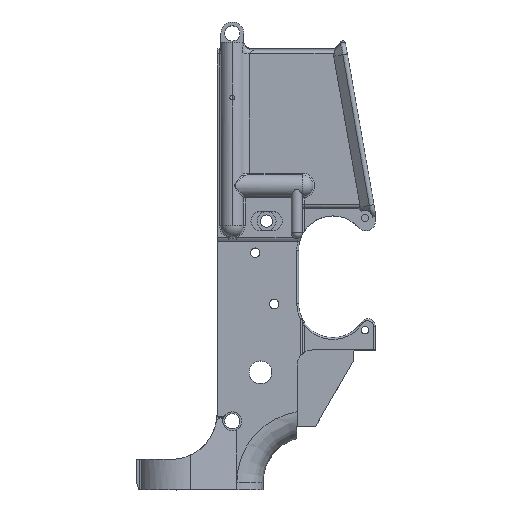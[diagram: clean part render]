
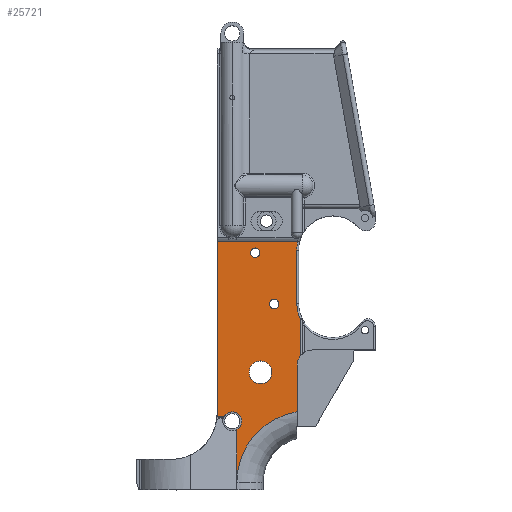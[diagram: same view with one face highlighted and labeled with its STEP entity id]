
A CAD part, top view. The second image highlights one B-rep face of the part: STEP entity #25721.
In plain terms, the highlighted planar face has unit normal (0, 0, 1).
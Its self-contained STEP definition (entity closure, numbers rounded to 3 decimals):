
#3836=CARTESIAN_POINT(' ',(0.033,-0.451,0.045));
#3837=VERTEX_POINT(' ',#3836);
#3926=CARTESIAN_POINT(' ',(0.033,-0.451,0.045));
#3931=DIRECTION(' ',(0.,1.,0.));
#3936=VECTOR(' ',#3931,1.);
#3941=LINE('',#3926,#3936);
#3946=CARTESIAN_POINT(' ',(0.033,-0.364,0.045));
#3947=VERTEX_POINT(' ',#3946);
#3951=EDGE_CURVE(' ',#3837,#3947,#3941,.T.);
#13861=CARTESIAN_POINT(' ',(0.,-0.338,0.045));
#13862=VERTEX_POINT(' ',#13861);
#13876=CARTESIAN_POINT(' ',(0.,-0.338,0.045));
#13881=DIRECTION(' ',(0.,1.,0.));
#13886=VECTOR(' ',#13881,1.);
#13891=LINE('',#13876,#13886);
#13896=CARTESIAN_POINT(' ',(0.,-0.055,0.045));
#13897=VERTEX_POINT(' ',#13896);
#13901=EDGE_CURVE(' ',#13862,#13897,#13891,.T.);
#17491=CARTESIAN_POINT(' ',(0.,-0.342,0.045));
#17492=VERTEX_POINT(' ',#17491);
#17506=CARTESIAN_POINT(' ',(-0.075,-0.338,0.045));
#17511=DIRECTION(' ',(0.,0.,1.));
#17516=DIRECTION(' ',(0.999,-0.053,0.));
#17521=AXIS2_PLACEMENT_3D(' ',#17506,#17511,#17516);
#17526=CIRCLE('',#17521,0.075);
#17531=EDGE_CURVE(' ',#17492,#13862,#17526,.T.);
#17851=CARTESIAN_POINT(' ',(0.041,-0.35,0.045));
#17852=VERTEX_POINT(' ',#17851);
#17866=CARTESIAN_POINT(' ',(0.025,-0.35,0.045));
#17871=DIRECTION(' ',(0.,0.,1.));
#17876=DIRECTION(' ',(1.,0.,0.));
#17881=AXIS2_PLACEMENT_3D(' ',#17866,#17871,#17876);
#17886=CIRCLE('',#17881,0.016);
#17891=CARTESIAN_POINT(' ',(0.011,-0.342,0.045));
#17892=VERTEX_POINT(' ',#17891);
#17896=EDGE_CURVE(' ',#17852,#17892,#17886,.T.);
#18146=CARTESIAN_POINT(' ',(0.025,-0.35,0.045));
#18151=DIRECTION(' ',(0.,0.,1.));
#18156=DIRECTION(' ',(0.481,-0.877,0.));
#18161=AXIS2_PLACEMENT_3D(' ',#18146,#18151,#18156);
#18166=CIRCLE('',#18161,0.016);
#18171=EDGE_CURVE(' ',#3947,#17852,#18166,.T.);
#24946=CARTESIAN_POINT(' ',(0.132,-0.334,0.045));
#24947=VERTEX_POINT(' ',#24946);
#24961=CARTESIAN_POINT(' ',(0.132,-0.334,0.045));
#24966=CARTESIAN_POINT(' ',(0.125,-0.336,0.045));
#24971=CARTESIAN_POINT(' ',(0.118,-0.337,0.045));
#24976=CARTESIAN_POINT(' ',(0.103,-0.342,0.045));
#24981=CARTESIAN_POINT(' ',(0.095,-0.347,0.045));
#24986=CARTESIAN_POINT(' ',(0.081,-0.355,0.045));
#24991=CARTESIAN_POINT(' ',(0.076,-0.359,0.045));
#24996=CARTESIAN_POINT(' ',(0.067,-0.367,0.045));
#25001=CARTESIAN_POINT(' ',(0.065,-0.37,0.045));
#25006=CARTESIAN_POINT(' ',(0.06,-0.375,0.045));
#25011=CARTESIAN_POINT(' ',(0.058,-0.377,0.045));
#25016=CARTESIAN_POINT(' ',(0.054,-0.382,0.045));
#25021=CARTESIAN_POINT(' ',(0.052,-0.385,0.045));
#25026=CARTESIAN_POINT(' ',(0.046,-0.396,0.045));
#25031=CARTESIAN_POINT(' ',(0.043,-0.402,0.045));
#25036=CARTESIAN_POINT(' ',(0.039,-0.412,0.045));
#25041=CARTESIAN_POINT(' ',(0.038,-0.416,0.045));
#25046=CARTESIAN_POINT(' ',(0.034,-0.43,0.045));
#25051=CARTESIAN_POINT(' ',(0.033,-0.435,0.045));
#25056=CARTESIAN_POINT(' ',(0.033,-0.442,0.045));
#25061=CARTESIAN_POINT(' ',(0.033,-0.445,0.045));
#25066=CARTESIAN_POINT(' ',(0.033,-0.451,0.045));
#25071=B_SPLINE_CURVE_WITH_KNOTS('',3,(#24961,#24966,#24971,#24976,#24981,#24986,#24991,#24996,#25001,#25006,#25011,#25016,#25021,#25026,#25031,#25036,#25041,#25046,#25051,#25056,#25061,#25066),.UNSPECIFIED.,.F.,.U.,(4,2,2,2,2,2,2,2,2,2,4),(0.,0.1,0.22,0.3,0.396,0.496,0.596,0.696,0.796,0.916,1.),.UNSPECIFIED.);
#25076=EDGE_CURVE(' ',#24947,#3837,#25071,.T.);
#25101=DIRECTION(' ',(0.,0.,1.));
#25106=CARTESIAN_POINT(' ',(0.,-0.451,0.045));
#25111=DIRECTION(' ',(1.,0.,0.));
#25116=AXIS2_PLACEMENT_3D(' ',#25106,#25101,#25111);
#25121=PLANE('',#25116);
#25126=ORIENTED_EDGE(' ',*,*,#17531,.F.);
#25131=CARTESIAN_POINT(' ',(0.,-0.342,0.045));
#25136=DIRECTION(' ',(0.997,-0.077,0.));
#25141=VECTOR(' ',#25136,1.);
#25146=LINE('',#25131,#25141);
#25151=EDGE_CURVE(' ',#17492,#17892,#25146,.T.);
#25156=ORIENTED_EDGE(' ',*,*,#25151,.T.);
#25161=ORIENTED_EDGE(' ',*,*,#17896,.F.);
#25166=ORIENTED_EDGE(' ',*,*,#18171,.F.);
#25171=ORIENTED_EDGE(' ',*,*,#3951,.F.);
#25176=ORIENTED_EDGE(' ',*,*,#25076,.F.);
#25181=CARTESIAN_POINT(' ',(0.132,-0.334,0.045));
#25186=DIRECTION(' ',(0.,1.,0.));
#25191=VECTOR(' ',#25186,1.);
#25196=LINE('',#25181,#25191);
#25201=CARTESIAN_POINT(' ',(0.132,-0.258,0.045));
#25202=VERTEX_POINT(' ',#25201);
#25206=EDGE_CURVE(' ',#24947,#25202,#25196,.T.);
#25211=ORIENTED_EDGE(' ',*,*,#25206,.T.);
#25216=CARTESIAN_POINT(' ',(0.157,-0.258,0.045));
#25221=DIRECTION(' ',(0.,0.,-1.));
#25226=DIRECTION(' ',(-1.,0.,0.));
#25231=AXIS2_PLACEMENT_3D(' ',#25216,#25221,#25226);
#25236=CIRCLE('',#25231,0.025);
#25241=CARTESIAN_POINT(' ',(0.137,-0.242,0.045));
#25242=VERTEX_POINT(' ',#25241);
#25246=EDGE_CURVE(' ',#25202,#25242,#25236,.T.);
#25251=ORIENTED_EDGE(' ',*,*,#25246,.T.);
#25256=CARTESIAN_POINT(' ',(0.137,-0.242,0.045));
#25261=DIRECTION(' ',(0.,1.,0.));
#25266=VECTOR(' ',#25261,1.);
#25271=LINE('',#25256,#25266);
#25276=CARTESIAN_POINT(' ',(0.137,-0.182,0.045));
#25277=VERTEX_POINT(' ',#25276);
#25281=EDGE_CURVE(' ',#25242,#25277,#25271,.T.);
#25286=ORIENTED_EDGE(' ',*,*,#25281,.T.);
#25291=CARTESIAN_POINT(' ',(0.19,-0.156,0.045));
#25296=DIRECTION(' ',(0.,0.,-1.));
#25301=DIRECTION(' ',(-0.899,-0.439,0.));
#25306=AXIS2_PLACEMENT_3D(' ',#25291,#25296,#25301);
#25311=CIRCLE('',#25306,0.059);
#25316=CARTESIAN_POINT(' ',(0.131,-0.156,0.045));
#25317=VERTEX_POINT(' ',#25316);
#25321=EDGE_CURVE(' ',#25277,#25317,#25311,.T.);
#25326=ORIENTED_EDGE(' ',*,*,#25321,.T.);
#25331=CARTESIAN_POINT(' ',(0.131,-0.156,0.045));
#25336=DIRECTION(' ',(0.,1.,0.));
#25341=VECTOR(' ',#25336,1.);
#25346=LINE('',#25331,#25341);
#25351=CARTESIAN_POINT(' ',(0.131,-0.069,0.045));
#25352=VERTEX_POINT(' ',#25351);
#25356=EDGE_CURVE(' ',#25317,#25352,#25346,.T.);
#25361=ORIENTED_EDGE(' ',*,*,#25356,.T.);
#25366=CARTESIAN_POINT(' ',(0.19,-0.069,0.045));
#25371=DIRECTION(' ',(0.,0.,-1.));
#25376=DIRECTION(' ',(-1.,0.,0.));
#25381=AXIS2_PLACEMENT_3D(' ',#25366,#25371,#25376);
#25386=CIRCLE('',#25381,0.059);
#25391=CARTESIAN_POINT(' ',(0.133,-0.055,0.045));
#25392=VERTEX_POINT(' ',#25391);
#25396=EDGE_CURVE(' ',#25352,#25392,#25386,.T.);
#25401=ORIENTED_EDGE(' ',*,*,#25396,.T.);
#25406=CARTESIAN_POINT(' ',(0.133,-0.055,0.045));
#25411=DIRECTION(' ',(-1.,0.,0.));
#25416=VECTOR(' ',#25411,1.);
#25421=LINE('',#25406,#25416);
#25426=EDGE_CURVE(' ',#25392,#13897,#25421,.T.);
#25431=ORIENTED_EDGE(' ',*,*,#25426,.T.);
#25436=ORIENTED_EDGE(' ',*,*,#13901,.F.);
#25441=EDGE_LOOP(' ',(#25126,#25156,#25161,#25166,#25171,#25176,#25211,#25251,#25286,#25326,#25361,#25401,#25431,#25436));
#25446=FACE_OUTER_BOUND(' ',#25441,.T.);
#25451=CARTESIAN_POINT(' ',(0.071,-0.27,0.045));
#25456=DIRECTION(' ',(0.,0.,-1.));
#25461=DIRECTION(' ',(1.,0.,0.));
#25466=AXIS2_PLACEMENT_3D(' ',#25451,#25456,#25461);
#25471=CIRCLE('',#25466,0.019);
#25476=CARTESIAN_POINT(' ',(0.09,-0.27,0.045));
#25477=VERTEX_POINT(' ',#25476);
#25481=CARTESIAN_POINT(' ',(0.053,-0.27,0.045));
#25482=VERTEX_POINT(' ',#25481);
#25486=EDGE_CURVE(' ',#25477,#25482,#25471,.T.);
#25491=ORIENTED_EDGE(' ',*,*,#25486,.T.);
#25496=CARTESIAN_POINT(' ',(0.071,-0.27,0.045));
#25501=DIRECTION(' ',(0.,-0.,-1.));
#25506=DIRECTION(' ',(-1.,0.,0.));
#25511=AXIS2_PLACEMENT_3D(' ',#25496,#25501,#25506);
#25516=CIRCLE('',#25511,0.019);
#25521=EDGE_CURVE(' ',#25482,#25477,#25516,.T.);
#25526=ORIENTED_EDGE(' ',*,*,#25521,.T.);
#25531=EDGE_LOOP(' ',(#25491,#25526));
#25536=FACE_BOUND(' ',#25531,.T.);
#25541=CARTESIAN_POINT(' ',(0.094,-0.157,0.045));
#25546=DIRECTION(' ',(0.,0.,-1.));
#25551=DIRECTION(' ',(1.,0.,0.));
#25556=AXIS2_PLACEMENT_3D(' ',#25541,#25546,#25551);
#25561=CIRCLE('',#25556,0.008);
#25566=CARTESIAN_POINT(' ',(0.102,-0.157,0.045));
#25567=VERTEX_POINT(' ',#25566);
#25571=CARTESIAN_POINT(' ',(0.086,-0.157,0.045));
#25572=VERTEX_POINT(' ',#25571);
#25576=EDGE_CURVE(' ',#25567,#25572,#25561,.T.);
#25581=ORIENTED_EDGE(' ',*,*,#25576,.T.);
#25586=CARTESIAN_POINT(' ',(0.094,-0.157,0.045));
#25591=DIRECTION(' ',(0.,0.,-1.));
#25596=DIRECTION(' ',(-1.,0.,0.));
#25601=AXIS2_PLACEMENT_3D(' ',#25586,#25591,#25596);
#25606=CIRCLE('',#25601,0.008);
#25611=EDGE_CURVE(' ',#25572,#25567,#25606,.T.);
#25616=ORIENTED_EDGE(' ',*,*,#25611,.T.);
#25621=EDGE_LOOP(' ',(#25581,#25616));
#25626=FACE_BOUND(' ',#25621,.T.);
#25631=CARTESIAN_POINT(' ',(0.063,-0.073,0.045));
#25636=DIRECTION(' ',(0.,0.,-1.));
#25641=DIRECTION(' ',(1.,0.,0.));
#25646=AXIS2_PLACEMENT_3D(' ',#25631,#25636,#25641);
#25651=CIRCLE('',#25646,0.008);
#25656=CARTESIAN_POINT(' ',(0.07,-0.073,0.045));
#25657=VERTEX_POINT(' ',#25656);
#25661=CARTESIAN_POINT(' ',(0.055,-0.073,0.045));
#25662=VERTEX_POINT(' ',#25661);
#25666=EDGE_CURVE(' ',#25657,#25662,#25651,.T.);
#25671=ORIENTED_EDGE(' ',*,*,#25666,.T.);
#25676=CARTESIAN_POINT(' ',(0.063,-0.073,0.045));
#25681=DIRECTION(' ',(0.,0.,-1.));
#25686=DIRECTION(' ',(-1.,0.,0.));
#25691=AXIS2_PLACEMENT_3D(' ',#25676,#25681,#25686);
#25696=CIRCLE('',#25691,0.008);
#25701=EDGE_CURVE(' ',#25662,#25657,#25696,.T.);
#25706=ORIENTED_EDGE(' ',*,*,#25701,.T.);
#25711=EDGE_LOOP(' ',(#25671,#25706));
#25716=FACE_BOUND(' ',#25711,.T.);
#25721=ADVANCED_FACE('',(#25446,#25536,#25626,#25716),#25121,.T.);
